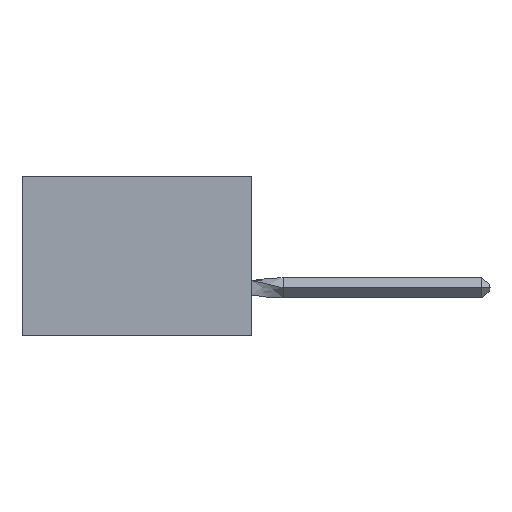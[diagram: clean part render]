
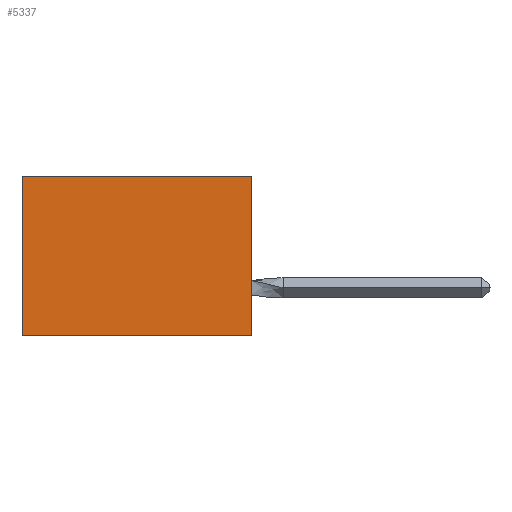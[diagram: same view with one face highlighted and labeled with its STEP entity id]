
A CAD part, left-side view. The second image highlights one B-rep face of the part: STEP entity #5337.
In plain terms, the highlighted planar face has unit normal (-1, 0, 0).
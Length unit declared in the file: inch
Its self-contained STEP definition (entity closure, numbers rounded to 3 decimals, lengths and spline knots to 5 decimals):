
#1346 = EDGE_CURVE ( 'NONE', #6403, #8145, #7321, .T. ) ;
#1542 = CARTESIAN_POINT ( 'NONE',  ( 0.305, 0., 0. ) ) ;
#1893 = CARTESIAN_POINT ( 'NONE',  ( 0.305, 0., -0.5 ) ) ;
#1936 = EDGE_LOOP ( 'NONE', ( #10208, #12718, #12426, #9382 ) ) ;
#2158 = DIRECTION ( 'NONE',  ( 1., 0., 0. ) ) ;
#2502 = AXIS2_PLACEMENT_3D ( 'NONE', #3405, #2158, #11274 ) ;
#2947 = EDGE_CURVE ( 'NONE', #12735, #6873, #5311, .T. ) ;
#3405 = CARTESIAN_POINT ( 'NONE',  ( 0.305, 0., -0.5 ) ) ;
#3958 = CARTESIAN_POINT ( 'NONE',  ( 0.305, 0., -0.5 ) ) ;
#4016 = CARTESIAN_POINT ( 'NONE',  ( 0.305, 0.72, -0.5 ) ) ;
#5311 = LINE ( 'NONE', #3958, #13445 ) ;
#5337 = ADVANCED_FACE ( 'NONE', ( #12664 ), #10142, .F. ) ;
#5587 = DIRECTION ( 'NONE',  ( 0., 0., -1. ) ) ;
#6403 = VERTEX_POINT ( 'NONE', #14461 ) ;
#6493 = CARTESIAN_POINT ( 'NONE',  ( 0.305, 0.72, 0. ) ) ;
#6873 = VERTEX_POINT ( 'NONE', #4016 ) ;
#7321 = LINE ( 'NONE', #1542, #12070 ) ;
#8145 = VERTEX_POINT ( 'NONE', #6493 ) ;
#8374 = VECTOR ( 'NONE', #9747, 39.37008 ) ;
#8735 = CARTESIAN_POINT ( 'NONE',  ( 0.305, 0., -0.5 ) ) ;
#9281 = LINE ( 'NONE', #13631, #11924 ) ;
#9382 = ORIENTED_EDGE ( 'NONE', *, *, #1346, .T. ) ;
#9478 = EDGE_CURVE ( 'NONE', #8145, #6873, #9281, .T. ) ;
#9747 = DIRECTION ( 'NONE',  ( 0., 0., -1. ) ) ;
#10142 = PLANE ( 'NONE',  #2502 ) ;
#10208 = ORIENTED_EDGE ( 'NONE', *, *, #9478, .T. ) ;
#11050 = EDGE_CURVE ( 'NONE', #6403, #12735, #14377, .T. ) ;
#11274 = DIRECTION ( 'NONE',  ( 0., 0., -1. ) ) ;
#11835 = DIRECTION ( 'NONE',  ( 0., 1., 0. ) ) ;
#11924 = VECTOR ( 'NONE', #5587, 39.37008 ) ;
#12070 = VECTOR ( 'NONE', #12794, 39.37008 ) ;
#12426 = ORIENTED_EDGE ( 'NONE', *, *, #11050, .F. ) ;
#12664 = FACE_OUTER_BOUND ( 'NONE', #1936, .T. ) ;
#12718 = ORIENTED_EDGE ( 'NONE', *, *, #2947, .F. ) ;
#12735 = VERTEX_POINT ( 'NONE', #8735 ) ;
#12794 = DIRECTION ( 'NONE',  ( 0., 1., 0. ) ) ;
#13445 = VECTOR ( 'NONE', #11835, 39.37008 ) ;
#13631 = CARTESIAN_POINT ( 'NONE',  ( 0.305, 0.72, -0.5 ) ) ;
#14377 = LINE ( 'NONE', #1893, #8374 ) ;
#14461 = CARTESIAN_POINT ( 'NONE',  ( 0.305, 0., 0. ) ) ;
